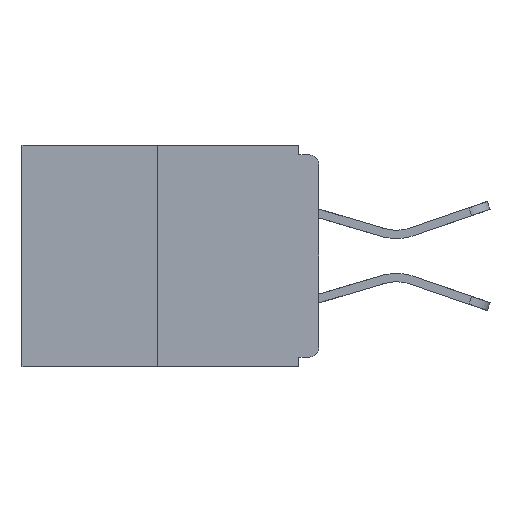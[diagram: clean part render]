
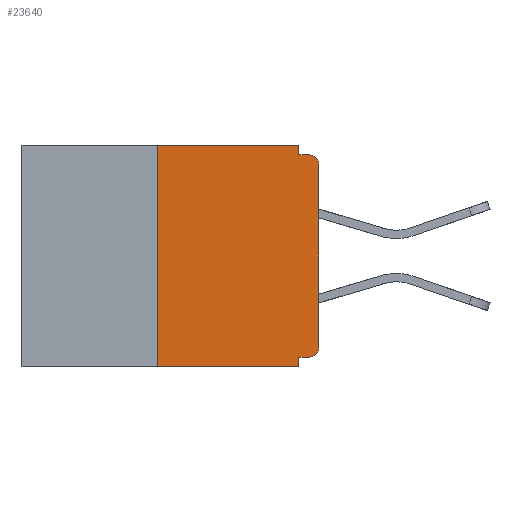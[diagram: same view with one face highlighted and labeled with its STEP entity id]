
A CAD part, left-side view. The second image highlights one B-rep face of the part: STEP entity #23640.
In plain terms, the highlighted planar face has unit normal (-1, 0, 0).
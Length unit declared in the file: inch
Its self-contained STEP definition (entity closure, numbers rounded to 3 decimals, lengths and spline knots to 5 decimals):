
#74 = LINE ( 'NONE', #983, #17921 ) ;
#655 = LINE ( 'NONE', #3071, #4866 ) ;
#793 = DIRECTION ( 'NONE',  ( 0., -1., 0. ) ) ;
#906 = LINE ( 'NONE', #21736, #7096 ) ;
#983 = CARTESIAN_POINT ( 'NONE',  ( 0., 0.031, -0.343 ) ) ;
#987 = DIRECTION ( 'NONE',  ( 0., 0., 1. ) ) ;
#1109 = ORIENTED_EDGE ( 'NONE', *, *, #5517, .F. ) ;
#1211 = CARTESIAN_POINT ( 'NONE',  ( 0., 0.015, -0.015 ) ) ;
#1550 = ORIENTED_EDGE ( 'NONE', *, *, #15337, .F. ) ;
#1875 = EDGE_CURVE ( 'NONE', #2032, #18106, #906, .T. ) ;
#2032 = VERTEX_POINT ( 'NONE', #10926 ) ;
#2515 = CARTESIAN_POINT ( 'NONE',  ( 0., 0., -0.03 ) ) ;
#2526 = DIRECTION ( 'NONE',  ( 0., 0., -1. ) ) ;
#2658 = EDGE_CURVE ( 'NONE', #18106, #9565, #12279, .T. ) ;
#2983 = ORIENTED_EDGE ( 'NONE', *, *, #21247, .F. ) ;
#3071 = CARTESIAN_POINT ( 'NONE',  ( 0., 0.25, 0. ) ) ;
#3321 = AXIS2_PLACEMENT_3D ( 'NONE', #10643, #17327, #11278 ) ;
#4261 = EDGE_CURVE ( 'NONE', #18388, #12220, #24768, .T. ) ;
#4336 = VERTEX_POINT ( 'NONE', #20947 ) ;
#4833 = CARTESIAN_POINT ( 'NONE',  ( 0., 0.015, -0.03 ) ) ;
#4866 = VECTOR ( 'NONE', #8995, 39.37008 ) ;
#5026 = VECTOR ( 'NONE', #24389, 39.37008 ) ;
#5117 = VERTEX_POINT ( 'NONE', #6591 ) ;
#5439 = DIRECTION ( 'NONE',  ( 0., -1., 0. ) ) ;
#5517 = EDGE_CURVE ( 'NONE', #16359, #17007, #21805, .T. ) ;
#6521 = ORIENTED_EDGE ( 'NONE', *, *, #20042, .F. ) ;
#6523 = CARTESIAN_POINT ( 'NONE',  ( 0., 0.031, -0.015 ) ) ;
#6540 = LINE ( 'NONE', #24173, #12093 ) ;
#6591 = CARTESIAN_POINT ( 'NONE',  ( 0., 0.25, 0. ) ) ;
#7096 = VECTOR ( 'NONE', #987, 39.37008 ) ;
#7332 = CARTESIAN_POINT ( 'NONE',  ( 0., 0.015, -0.328 ) ) ;
#8995 = DIRECTION ( 'NONE',  ( 0., 0., 1. ) ) ;
#9438 = PLANE ( 'NONE',  #22217 ) ;
#9481 = VECTOR ( 'NONE', #793, 39.37008 ) ;
#9565 = VERTEX_POINT ( 'NONE', #1211 ) ;
#10405 = EDGE_CURVE ( 'NONE', #15201, #4336, #21562, .T. ) ;
#10643 = CARTESIAN_POINT ( 'NONE',  ( 0., 0.015, -0.313 ) ) ;
#10926 = CARTESIAN_POINT ( 'NONE',  ( 0., 0., -0.313 ) ) ;
#11221 = AXIS2_PLACEMENT_3D ( 'NONE', #4833, #21420, #2526 ) ;
#11278 = DIRECTION ( 'NONE',  ( 0., 0., -1. ) ) ;
#12093 = VECTOR ( 'NONE', #5439, 39.37008 ) ;
#12220 = VERTEX_POINT ( 'NONE', #6523 ) ;
#12279 = CIRCLE ( 'NONE', #11221, 0.015 ) ;
#12721 = ORIENTED_EDGE ( 'NONE', *, *, #1875, .T. ) ;
#12730 = ORIENTED_EDGE ( 'NONE', *, *, #2658, .T. ) ;
#13241 = EDGE_CURVE ( 'NONE', #16359, #2032, #13493, .T. ) ;
#13467 = DIRECTION ( 'NONE',  ( 0., 0., -1. ) ) ;
#13493 = CIRCLE ( 'NONE', #3321, 0.015 ) ;
#14969 = ORIENTED_EDGE ( 'NONE', *, *, #13241, .T. ) ;
#15201 = VERTEX_POINT ( 'NONE', #25208 ) ;
#15296 = EDGE_CURVE ( 'NONE', #15201, #5117, #655, .T. ) ;
#15337 = EDGE_CURVE ( 'NONE', #12220, #9565, #20447, .T. ) ;
#15530 = FACE_OUTER_BOUND ( 'NONE', #26059, .T. ) ;
#15681 = CARTESIAN_POINT ( 'NONE',  ( 0., 0.46, 0. ) ) ;
#15849 = ORIENTED_EDGE ( 'NONE', *, *, #4261, .F. ) ;
#16026 = DIRECTION ( 'NONE',  ( 1., 0., 0. ) ) ;
#16334 = VECTOR ( 'NONE', #22580, 39.37008 ) ;
#16359 = VERTEX_POINT ( 'NONE', #7332 ) ;
#16374 = VECTOR ( 'NONE', #22478, 39.37008 ) ;
#16868 = CARTESIAN_POINT ( 'NONE',  ( 0., 0.031, -0.328 ) ) ;
#17007 = VERTEX_POINT ( 'NONE', #16868 ) ;
#17033 = ORIENTED_EDGE ( 'NONE', *, *, #15296, .F. ) ;
#17327 = DIRECTION ( 'NONE',  ( -1., 0., 0. ) ) ;
#17921 = VECTOR ( 'NONE', #13467, 39.37008 ) ;
#18106 = VERTEX_POINT ( 'NONE', #2515 ) ;
#18346 = CARTESIAN_POINT ( 'NONE',  ( 0., 0.46, -0.343 ) ) ;
#18388 = VERTEX_POINT ( 'NONE', #25896 ) ;
#19736 = ORIENTED_EDGE ( 'NONE', *, *, #10405, .T. ) ;
#20042 = EDGE_CURVE ( 'NONE', #17007, #4336, #74, .T. ) ;
#20447 = LINE ( 'NONE', #25663, #9481 ) ;
#20947 = CARTESIAN_POINT ( 'NONE',  ( 0., 0.031, -0.343 ) ) ;
#21247 = EDGE_CURVE ( 'NONE', #5117, #18388, #6540, .T. ) ;
#21420 = DIRECTION ( 'NONE',  ( -1., 0., 0. ) ) ;
#21562 = LINE ( 'NONE', #18346, #5026 ) ;
#21736 = CARTESIAN_POINT ( 'NONE',  ( 0., 0., 0. ) ) ;
#21805 = LINE ( 'NONE', #24685, #16334 ) ;
#22217 = AXIS2_PLACEMENT_3D ( 'NONE', #15681, #16026, #24230 ) ;
#22478 = DIRECTION ( 'NONE',  ( 0., 0., -1. ) ) ;
#22580 = DIRECTION ( 'NONE',  ( 0., 1., 0. ) ) ;
#23640 = ADVANCED_FACE ( 'NONE', ( #15530 ), #9438, .F. ) ;
#24173 = CARTESIAN_POINT ( 'NONE',  ( 0., 0.46, 0. ) ) ;
#24230 = DIRECTION ( 'NONE',  ( 0., 0., -1. ) ) ;
#24389 = DIRECTION ( 'NONE',  ( 0., -1., 0. ) ) ;
#24685 = CARTESIAN_POINT ( 'NONE',  ( 0., 0., -0.328 ) ) ;
#24764 = CARTESIAN_POINT ( 'NONE',  ( 0., 0.031, 0. ) ) ;
#24768 = LINE ( 'NONE', #24764, #16374 ) ;
#25208 = CARTESIAN_POINT ( 'NONE',  ( 0., 0.25, -0.343 ) ) ;
#25663 = CARTESIAN_POINT ( 'NONE',  ( 0., 0., -0.015 ) ) ;
#25896 = CARTESIAN_POINT ( 'NONE',  ( 0., 0.031, 0. ) ) ;
#26059 = EDGE_LOOP ( 'NONE', ( #2983, #17033, #19736, #6521, #1109, #14969, #12721, #12730, #1550, #15849 ) ) ;
